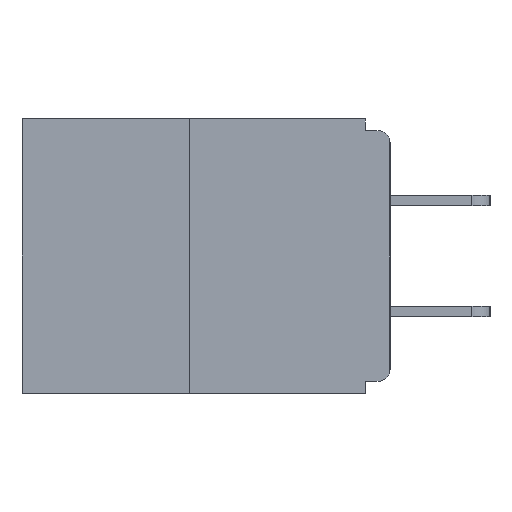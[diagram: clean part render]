
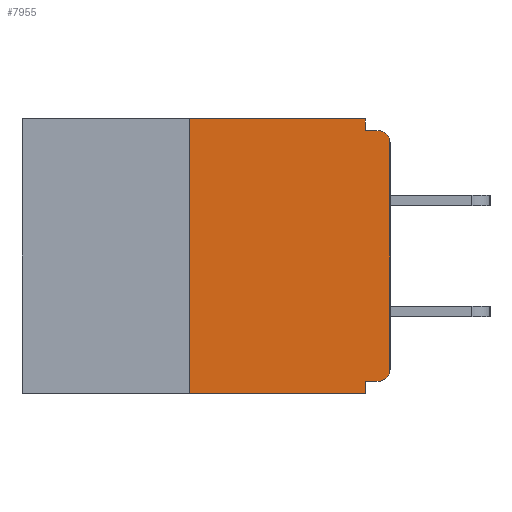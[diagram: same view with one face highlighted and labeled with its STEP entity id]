
A CAD part, left-side view. The second image highlights one B-rep face of the part: STEP entity #7955.
In plain terms, the highlighted planar face has unit normal (-1, 0, 0).
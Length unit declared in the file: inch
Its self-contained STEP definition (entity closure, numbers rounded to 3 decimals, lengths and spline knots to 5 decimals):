
#135 = CIRCLE ( 'NONE', #11504, 0.015 ) ;
#178 = ORIENTED_EDGE ( 'NONE', *, *, #9957, .F. ) ;
#286 = ORIENTED_EDGE ( 'NONE', *, *, #3502, .F. ) ;
#634 = CARTESIAN_POINT ( 'NONE',  ( 0., 0., -0.015 ) ) ;
#641 = DIRECTION ( 'NONE',  ( 0., 0., -1. ) ) ;
#764 = VERTEX_POINT ( 'NONE', #8205 ) ;
#1160 = VECTOR ( 'NONE', #8164, 39.37008 ) ;
#1202 = DIRECTION ( 'NONE',  ( 0., 0., -1. ) ) ;
#1561 = CIRCLE ( 'NONE', #6019, 0.015 ) ;
#1671 = LINE ( 'NONE', #5068, #17921 ) ;
#2402 = CARTESIAN_POINT ( 'NONE',  ( 0., 0.46, 0. ) ) ;
#2603 = VECTOR ( 'NONE', #3718, 39.37008 ) ;
#2750 = ORIENTED_EDGE ( 'NONE', *, *, #14435, .F. ) ;
#2976 = VERTEX_POINT ( 'NONE', #9303 ) ;
#2996 = VERTEX_POINT ( 'NONE', #7967 ) ;
#3397 = VERTEX_POINT ( 'NONE', #7236 ) ;
#3453 = DIRECTION ( 'NONE',  ( 0., -1., 0. ) ) ;
#3463 = CARTESIAN_POINT ( 'NONE',  ( 0., 0.46, 0. ) ) ;
#3502 = EDGE_CURVE ( 'NONE', #764, #15831, #8442, .T. ) ;
#3718 = DIRECTION ( 'NONE',  ( 0., -1., 0. ) ) ;
#3740 = CARTESIAN_POINT ( 'NONE',  ( 0., 0., -0.313 ) ) ;
#3856 = VERTEX_POINT ( 'NONE', #13683 ) ;
#3897 = VERTEX_POINT ( 'NONE', #12438 ) ;
#3904 = DIRECTION ( 'NONE',  ( -1., 0., 0. ) ) ;
#4531 = DIRECTION ( 'NONE',  ( 0., 0., -1. ) ) ;
#4712 = EDGE_CURVE ( 'NONE', #14743, #2976, #10691, .T. ) ;
#4777 = CARTESIAN_POINT ( 'NONE',  ( 0., 0.015, -0.03 ) ) ;
#5068 = CARTESIAN_POINT ( 'NONE',  ( 0., 0., 0. ) ) ;
#5470 = DIRECTION ( 'NONE',  ( 0., 0., -1. ) ) ;
#6019 = AXIS2_PLACEMENT_3D ( 'NONE', #8413, #3904, #1202 ) ;
#6044 = ORIENTED_EDGE ( 'NONE', *, *, #13491, .F. ) ;
#6232 = DIRECTION ( 'NONE',  ( -1., 0., 0. ) ) ;
#6652 = VECTOR ( 'NONE', #5470, 39.37008 ) ;
#7214 = EDGE_CURVE ( 'NONE', #3897, #10708, #1561, .T. ) ;
#7236 = CARTESIAN_POINT ( 'NONE',  ( 0., 0.031, -0.343 ) ) ;
#7493 = VECTOR ( 'NONE', #10124, 39.37008 ) ;
#7574 = VERTEX_POINT ( 'NONE', #10128 ) ;
#7939 = ORIENTED_EDGE ( 'NONE', *, *, #4712, .F. ) ;
#7955 = ADVANCED_FACE ( 'NONE', ( #13513 ), #16534, .F. ) ;
#7967 = CARTESIAN_POINT ( 'NONE',  ( 0., 0.031, -0.328 ) ) ;
#8145 = ORIENTED_EDGE ( 'NONE', *, *, #7214, .T. ) ;
#8164 = DIRECTION ( 'NONE',  ( 0., -1., 0. ) ) ;
#8199 = VECTOR ( 'NONE', #4531, 39.37008 ) ;
#8205 = CARTESIAN_POINT ( 'NONE',  ( 0., 0.031, -0.015 ) ) ;
#8413 = CARTESIAN_POINT ( 'NONE',  ( 0., 0.015, -0.313 ) ) ;
#8442 = LINE ( 'NONE', #634, #11150 ) ;
#9303 = CARTESIAN_POINT ( 'NONE',  ( 0., 0.25, 0. ) ) ;
#9322 = EDGE_CURVE ( 'NONE', #14743, #3397, #9409, .T. ) ;
#9409 = LINE ( 'NONE', #13326, #2603 ) ;
#9957 = EDGE_CURVE ( 'NONE', #2996, #3397, #11636, .T. ) ;
#10124 = DIRECTION ( 'NONE',  ( 0., 0., 1. ) ) ;
#10128 = CARTESIAN_POINT ( 'NONE',  ( 0., 0.031, 0. ) ) ;
#10389 = CARTESIAN_POINT ( 'NONE',  ( 0., 0.031, 0. ) ) ;
#10512 = EDGE_CURVE ( 'NONE', #3897, #2996, #16796, .T. ) ;
#10691 = LINE ( 'NONE', #15900, #7493 ) ;
#10708 = VERTEX_POINT ( 'NONE', #3740 ) ;
#11090 = DIRECTION ( 'NONE',  ( 0., 0., 1. ) ) ;
#11150 = VECTOR ( 'NONE', #3453, 39.37008 ) ;
#11504 = AXIS2_PLACEMENT_3D ( 'NONE', #4777, #6232, #14902 ) ;
#11636 = LINE ( 'NONE', #16428, #6652 ) ;
#11898 = CARTESIAN_POINT ( 'NONE',  ( 0., 0.25, -0.343 ) ) ;
#11998 = ORIENTED_EDGE ( 'NONE', *, *, #17503, .T. ) ;
#12048 = EDGE_LOOP ( 'NONE', ( #2750, #7939, #18549, #178, #18685, #8145, #18503, #11998, #286, #6044 ) ) ;
#12344 = DIRECTION ( 'NONE',  ( 0., 1., 0. ) ) ;
#12438 = CARTESIAN_POINT ( 'NONE',  ( 0., 0.015, -0.328 ) ) ;
#13035 = CARTESIAN_POINT ( 'NONE',  ( 0., 0.015, -0.015 ) ) ;
#13107 = EDGE_CURVE ( 'NONE', #10708, #3856, #1671, .T. ) ;
#13326 = CARTESIAN_POINT ( 'NONE',  ( 0., 0.46, -0.343 ) ) ;
#13491 = EDGE_CURVE ( 'NONE', #7574, #764, #17437, .T. ) ;
#13507 = DIRECTION ( 'NONE',  ( 1., 0., 0. ) ) ;
#13513 = FACE_OUTER_BOUND ( 'NONE', #12048, .T. ) ;
#13683 = CARTESIAN_POINT ( 'NONE',  ( 0., 0., -0.03 ) ) ;
#14435 = EDGE_CURVE ( 'NONE', #2976, #7574, #17634, .T. ) ;
#14743 = VERTEX_POINT ( 'NONE', #11898 ) ;
#14902 = DIRECTION ( 'NONE',  ( 0., 0., -1. ) ) ;
#15831 = VERTEX_POINT ( 'NONE', #13035 ) ;
#15900 = CARTESIAN_POINT ( 'NONE',  ( 0., 0.25, 0. ) ) ;
#16428 = CARTESIAN_POINT ( 'NONE',  ( 0., 0.031, -0.343 ) ) ;
#16534 = PLANE ( 'NONE',  #17036 ) ;
#16582 = VECTOR ( 'NONE', #12344, 39.37008 ) ;
#16796 = LINE ( 'NONE', #17867, #16582 ) ;
#17036 = AXIS2_PLACEMENT_3D ( 'NONE', #3463, #13507, #641 ) ;
#17437 = LINE ( 'NONE', #10389, #8199 ) ;
#17503 = EDGE_CURVE ( 'NONE', #3856, #15831, #135, .T. ) ;
#17634 = LINE ( 'NONE', #2402, #1160 ) ;
#17867 = CARTESIAN_POINT ( 'NONE',  ( 0., 0., -0.328 ) ) ;
#17921 = VECTOR ( 'NONE', #11090, 39.37008 ) ;
#18503 = ORIENTED_EDGE ( 'NONE', *, *, #13107, .T. ) ;
#18549 = ORIENTED_EDGE ( 'NONE', *, *, #9322, .T. ) ;
#18685 = ORIENTED_EDGE ( 'NONE', *, *, #10512, .F. ) ;
